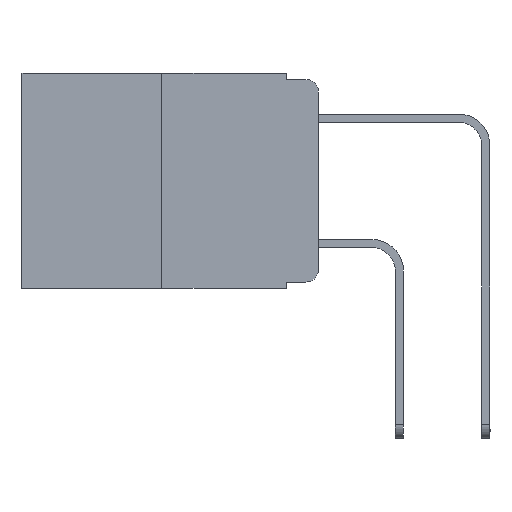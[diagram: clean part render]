
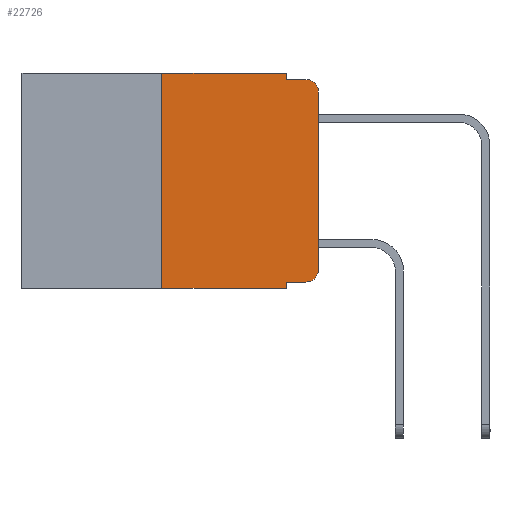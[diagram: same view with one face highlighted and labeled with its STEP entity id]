
A CAD part, left-side view. The second image highlights one B-rep face of the part: STEP entity #22726.
In plain terms, the highlighted planar face has unit normal (-1, 0, 0).
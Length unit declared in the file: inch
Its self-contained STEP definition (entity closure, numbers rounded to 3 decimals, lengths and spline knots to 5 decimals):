
#188 = EDGE_CURVE ( 'NONE', #23625, #2309, #13876, .T. ) ;
#528 = VECTOR ( 'NONE', #8987, 39.37008 ) ;
#690 = PLANE ( 'NONE',  #19779 ) ;
#909 = VECTOR ( 'NONE', #9817, 39.37008 ) ;
#1180 = VERTEX_POINT ( 'NONE', #7388 ) ;
#2015 = VECTOR ( 'NONE', #9822, 39.37008 ) ;
#2103 = CARTESIAN_POINT ( 'NONE',  ( 0., 0.051, -0.01 ) ) ;
#2309 = VERTEX_POINT ( 'NONE', #23827 ) ;
#2949 = EDGE_CURVE ( 'NONE', #17688, #1180, #9164, .T. ) ;
#3202 = CARTESIAN_POINT ( 'NONE',  ( 0., 0., -0.03 ) ) ;
#3353 = CIRCLE ( 'NONE', #7942, 0.02 ) ;
#3407 = EDGE_CURVE ( 'NONE', #17219, #9315, #3353, .T. ) ;
#3521 = VERTEX_POINT ( 'NONE', #21787 ) ;
#4846 = LINE ( 'NONE', #17888, #14815 ) ;
#4858 = EDGE_CURVE ( 'NONE', #8424, #17046, #17653, .T. ) ;
#5382 = VECTOR ( 'NONE', #22222, 39.37008 ) ;
#5556 = ORIENTED_EDGE ( 'NONE', *, *, #7268, .F. ) ;
#6170 = CARTESIAN_POINT ( 'NONE',  ( 0., 0.473, 0. ) ) ;
#6429 = ORIENTED_EDGE ( 'NONE', *, *, #11764, .T. ) ;
#6705 = DIRECTION ( 'NONE',  ( 0., -1., 0. ) ) ;
#6831 = CARTESIAN_POINT ( 'NONE',  ( 0., 0.02, -0.313 ) ) ;
#7268 = EDGE_CURVE ( 'NONE', #3521, #1180, #15451, .T. ) ;
#7287 = ORIENTED_EDGE ( 'NONE', *, *, #4858, .F. ) ;
#7388 = CARTESIAN_POINT ( 'NONE',  ( 0., 0.051, -0.343 ) ) ;
#7681 = CARTESIAN_POINT ( 'NONE',  ( 0., 0.02, -0.03 ) ) ;
#7828 = ORIENTED_EDGE ( 'NONE', *, *, #18449, .F. ) ;
#7942 = AXIS2_PLACEMENT_3D ( 'NONE', #6831, #23731, #10735 ) ;
#8414 = LINE ( 'NONE', #20112, #22254 ) ;
#8424 = VERTEX_POINT ( 'NONE', #15741 ) ;
#8469 = EDGE_LOOP ( 'NONE', ( #6429, #9656, #8763, #19475, #7287, #7828, #21441, #5556, #17165, #20220 ) ) ;
#8763 = ORIENTED_EDGE ( 'NONE', *, *, #14849, .F. ) ;
#8987 = DIRECTION ( 'NONE',  ( 0., 0., 1. ) ) ;
#9164 = LINE ( 'NONE', #20435, #5382 ) ;
#9315 = VERTEX_POINT ( 'NONE', #14306 ) ;
#9656 = ORIENTED_EDGE ( 'NONE', *, *, #188, .T. ) ;
#9817 = DIRECTION ( 'NONE',  ( 0., -1., 0. ) ) ;
#9822 = DIRECTION ( 'NONE',  ( 0., 0., -1. ) ) ;
#10008 = VECTOR ( 'NONE', #22527, 39.37008 ) ;
#10735 = DIRECTION ( 'NONE',  ( 0., 0., -1. ) ) ;
#10871 = LINE ( 'NONE', #2103, #10008 ) ;
#11600 = DIRECTION ( 'NONE',  ( -1., 0., 0. ) ) ;
#11715 = DIRECTION ( 'NONE',  ( 0., 0., -1. ) ) ;
#11764 = EDGE_CURVE ( 'NONE', #9315, #23625, #8414, .T. ) ;
#12626 = DIRECTION ( 'NONE',  ( 0., 0., 1. ) ) ;
#13398 = VECTOR ( 'NONE', #19763, 39.37008 ) ;
#13509 = DIRECTION ( 'NONE',  ( 0., 0., -1. ) ) ;
#13848 = CARTESIAN_POINT ( 'NONE',  ( 0., 0.473, 0. ) ) ;
#13876 = CIRCLE ( 'NONE', #23468, 0.02 ) ;
#14306 = CARTESIAN_POINT ( 'NONE',  ( 0., 0., -0.313 ) ) ;
#14815 = VECTOR ( 'NONE', #6705, 39.37008 ) ;
#14849 = EDGE_CURVE ( 'NONE', #20927, #2309, #10871, .T. ) ;
#15451 = LINE ( 'NONE', #21486, #13398 ) ;
#15539 = CARTESIAN_POINT ( 'NONE',  ( 0., 0.02, -0.333 ) ) ;
#15624 = CARTESIAN_POINT ( 'NONE',  ( 0., 0.051, 0. ) ) ;
#15741 = CARTESIAN_POINT ( 'NONE',  ( 0., 0.25, 0. ) ) ;
#16660 = LINE ( 'NONE', #17510, #2015 ) ;
#17046 = VERTEX_POINT ( 'NONE', #15624 ) ;
#17165 = ORIENTED_EDGE ( 'NONE', *, *, #22969, .T. ) ;
#17219 = VERTEX_POINT ( 'NONE', #15539 ) ;
#17429 = DIRECTION ( 'NONE',  ( 1., 0., 0. ) ) ;
#17510 = CARTESIAN_POINT ( 'NONE',  ( 0., 0.051, 0. ) ) ;
#17653 = LINE ( 'NONE', #13848, #909 ) ;
#17688 = VERTEX_POINT ( 'NONE', #21357 ) ;
#17843 = EDGE_CURVE ( 'NONE', #17046, #20927, #16660, .T. ) ;
#17888 = CARTESIAN_POINT ( 'NONE',  ( 0., 0.051, -0.333 ) ) ;
#18236 = CARTESIAN_POINT ( 'NONE',  ( 0., 0.25, 0. ) ) ;
#18449 = EDGE_CURVE ( 'NONE', #17688, #8424, #19574, .T. ) ;
#18689 = FACE_OUTER_BOUND ( 'NONE', #8469, .T. ) ;
#19475 = ORIENTED_EDGE ( 'NONE', *, *, #17843, .F. ) ;
#19574 = LINE ( 'NONE', #18236, #528 ) ;
#19763 = DIRECTION ( 'NONE',  ( 0., 0., -1. ) ) ;
#19779 = AXIS2_PLACEMENT_3D ( 'NONE', #6170, #17429, #11715 ) ;
#20112 = CARTESIAN_POINT ( 'NONE',  ( 0., 0., 0. ) ) ;
#20136 = CARTESIAN_POINT ( 'NONE',  ( 0., 0.051, -0.01 ) ) ;
#20220 = ORIENTED_EDGE ( 'NONE', *, *, #3407, .T. ) ;
#20435 = CARTESIAN_POINT ( 'NONE',  ( 0., 0.473, -0.343 ) ) ;
#20927 = VERTEX_POINT ( 'NONE', #20136 ) ;
#21357 = CARTESIAN_POINT ( 'NONE',  ( 0., 0.25, -0.343 ) ) ;
#21441 = ORIENTED_EDGE ( 'NONE', *, *, #2949, .T. ) ;
#21486 = CARTESIAN_POINT ( 'NONE',  ( 0., 0.051, 0. ) ) ;
#21787 = CARTESIAN_POINT ( 'NONE',  ( 0., 0.051, -0.333 ) ) ;
#22222 = DIRECTION ( 'NONE',  ( 0., -1., 0. ) ) ;
#22254 = VECTOR ( 'NONE', #12626, 39.37008 ) ;
#22527 = DIRECTION ( 'NONE',  ( 0., -1., 0. ) ) ;
#22726 = ADVANCED_FACE ( 'NONE', ( #18689 ), #690, .F. ) ;
#22969 = EDGE_CURVE ( 'NONE', #3521, #17219, #4846, .T. ) ;
#23468 = AXIS2_PLACEMENT_3D ( 'NONE', #7681, #11600, #13509 ) ;
#23625 = VERTEX_POINT ( 'NONE', #3202 ) ;
#23731 = DIRECTION ( 'NONE',  ( -1., 0., 0. ) ) ;
#23827 = CARTESIAN_POINT ( 'NONE',  ( 0., 0.02, -0.01 ) ) ;
